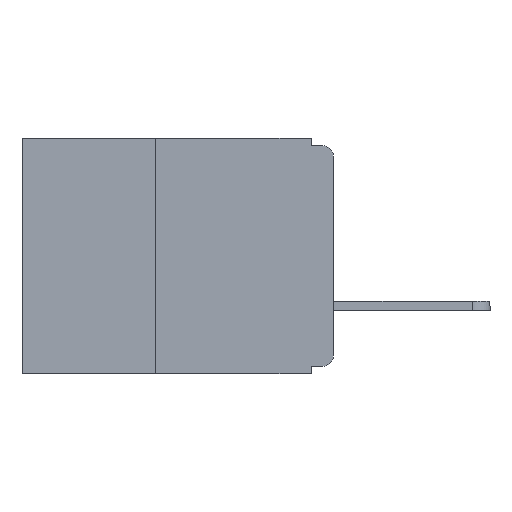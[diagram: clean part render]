
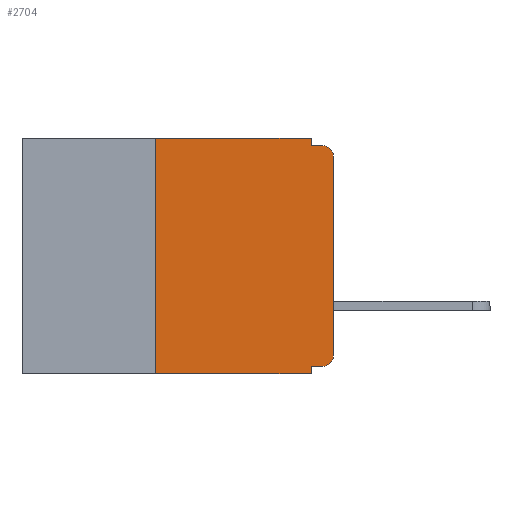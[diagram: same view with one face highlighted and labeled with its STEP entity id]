
A CAD part, left-side view. The second image highlights one B-rep face of the part: STEP entity #2704.
In plain terms, the highlighted planar face has unit normal (-1, 0, 0).
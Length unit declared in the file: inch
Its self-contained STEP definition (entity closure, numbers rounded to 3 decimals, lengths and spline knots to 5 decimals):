
#393 = ORIENTED_EDGE ( 'NONE', *, *, #2934, .F. ) ;
#670 = CARTESIAN_POINT ( 'NONE',  ( 0., 0., -0.01 ) ) ;
#1134 = CARTESIAN_POINT ( 'NONE',  ( 0., 0.437, -0.33 ) ) ;
#1519 = LINE ( 'NONE', #21604, #22971 ) ;
#2468 = DIRECTION ( 'NONE',  ( 0., 0., -1. ) ) ;
#2632 = LINE ( 'NONE', #20486, #23436 ) ;
#2704 = ADVANCED_FACE ( 'NONE', ( #4771 ), #10518, .F. ) ;
#2796 = DIRECTION ( 'NONE',  ( 0., -1., 0. ) ) ;
#2934 = EDGE_CURVE ( 'NONE', #14700, #11044, #10099, .T. ) ;
#3012 = ORIENTED_EDGE ( 'NONE', *, *, #5833, .F. ) ;
#3144 = DIRECTION ( 'NONE',  ( -1., 0., 0. ) ) ;
#3207 = CARTESIAN_POINT ( 'NONE',  ( 0., 0.031, -0.33 ) ) ;
#3247 = CARTESIAN_POINT ( 'NONE',  ( 0., 0.031, -0.33 ) ) ;
#3608 = DIRECTION ( 'NONE',  ( 0., 0., -1. ) ) ;
#3685 = CARTESIAN_POINT ( 'NONE',  ( 0., 0.031, 0. ) ) ;
#4215 = CARTESIAN_POINT ( 'NONE',  ( 0., 0.437, 0. ) ) ;
#4442 = VECTOR ( 'NONE', #2468, 39.37008 ) ;
#4647 = ORIENTED_EDGE ( 'NONE', *, *, #9009, .F. ) ;
#4750 = EDGE_CURVE ( 'NONE', #20204, #13691, #24163, .T. ) ;
#4771 = FACE_OUTER_BOUND ( 'NONE', #12851, .T. ) ;
#4803 = AXIS2_PLACEMENT_3D ( 'NONE', #15691, #3144, #17779 ) ;
#4807 = LINE ( 'NONE', #1134, #20767 ) ;
#4853 = VECTOR ( 'NONE', #2796, 39.37008 ) ;
#5833 = EDGE_CURVE ( 'NONE', #7580, #12090, #25761, .T. ) ;
#6058 = CARTESIAN_POINT ( 'NONE',  ( 0., 0.25, 0. ) ) ;
#6938 = EDGE_CURVE ( 'NONE', #25751, #11863, #2632, .T. ) ;
#7128 = DIRECTION ( 'NONE',  ( 0., -1., 0. ) ) ;
#7425 = LINE ( 'NONE', #24303, #12403 ) ;
#7580 = VERTEX_POINT ( 'NONE', #18480 ) ;
#7639 = ORIENTED_EDGE ( 'NONE', *, *, #6938, .F. ) ;
#8133 = AXIS2_PLACEMENT_3D ( 'NONE', #18391, #18327, #18323 ) ;
#8964 = ORIENTED_EDGE ( 'NONE', *, *, #17794, .T. ) ;
#9009 = EDGE_CURVE ( 'NONE', #12090, #13691, #21423, .T. ) ;
#9742 = DIRECTION ( 'NONE',  ( 0., 0., 1. ) ) ;
#10099 = LINE ( 'NONE', #3207, #4442 ) ;
#10230 = DIRECTION ( 'NONE',  ( 0., 0., 1. ) ) ;
#10518 = PLANE ( 'NONE',  #23278 ) ;
#10558 = CARTESIAN_POINT ( 'NONE',  ( 0., 0.25, -0.33 ) ) ;
#11044 = VERTEX_POINT ( 'NONE', #3247 ) ;
#11780 = CARTESIAN_POINT ( 'NONE',  ( 0., 0., 0. ) ) ;
#11863 = VERTEX_POINT ( 'NONE', #6058 ) ;
#12090 = VERTEX_POINT ( 'NONE', #20936 ) ;
#12304 = EDGE_CURVE ( 'NONE', #11863, #7580, #1519, .T. ) ;
#12403 = VECTOR ( 'NONE', #26367, 39.37008 ) ;
#12510 = EDGE_CURVE ( 'NONE', #17296, #14700, #7425, .T. ) ;
#12851 = EDGE_LOOP ( 'NONE', ( #24116, #19972, #4647, #3012, #17442, #7639, #8964, #393, #17760, #23195 ) ) ;
#13691 = VERTEX_POINT ( 'NONE', #20226 ) ;
#14700 = VERTEX_POINT ( 'NONE', #21886 ) ;
#15691 = CARTESIAN_POINT ( 'NONE',  ( 0., 0.015, -0.305 ) ) ;
#17296 = VERTEX_POINT ( 'NONE', #20790 ) ;
#17442 = ORIENTED_EDGE ( 'NONE', *, *, #12304, .F. ) ;
#17759 = EDGE_CURVE ( 'NONE', #17296, #26332, #21386, .T. ) ;
#17760 = ORIENTED_EDGE ( 'NONE', *, *, #12510, .F. ) ;
#17779 = DIRECTION ( 'NONE',  ( 0., 0., -1. ) ) ;
#17794 = EDGE_CURVE ( 'NONE', #25751, #11044, #4807, .T. ) ;
#17869 = DIRECTION ( 'NONE',  ( 0., -1., 0. ) ) ;
#18323 = DIRECTION ( 'NONE',  ( 0., 0., -1. ) ) ;
#18327 = DIRECTION ( 'NONE',  ( -1., 0., 0. ) ) ;
#18391 = CARTESIAN_POINT ( 'NONE',  ( 0., 0.015, -0.025 ) ) ;
#18447 = VECTOR ( 'NONE', #9742, 39.37008 ) ;
#18480 = CARTESIAN_POINT ( 'NONE',  ( 0., 0.031, 0. ) ) ;
#19667 = VECTOR ( 'NONE', #3608, 39.37008 ) ;
#19972 = ORIENTED_EDGE ( 'NONE', *, *, #4750, .T. ) ;
#20204 = VERTEX_POINT ( 'NONE', #26069 ) ;
#20226 = CARTESIAN_POINT ( 'NONE',  ( 0., 0.015, -0.01 ) ) ;
#20486 = CARTESIAN_POINT ( 'NONE',  ( 0., 0.25, -0.33 ) ) ;
#20767 = VECTOR ( 'NONE', #17869, 39.37008 ) ;
#20790 = CARTESIAN_POINT ( 'NONE',  ( 0., 0.015, -0.32 ) ) ;
#20936 = CARTESIAN_POINT ( 'NONE',  ( 0., 0.031, -0.01 ) ) ;
#21386 = CIRCLE ( 'NONE', #4803, 0.015 ) ;
#21423 = LINE ( 'NONE', #670, #4853 ) ;
#21604 = CARTESIAN_POINT ( 'NONE',  ( 0., 0.437, 0. ) ) ;
#21886 = CARTESIAN_POINT ( 'NONE',  ( 0., 0.031, -0.32 ) ) ;
#22971 = VECTOR ( 'NONE', #7128, 39.37008 ) ;
#23076 = CARTESIAN_POINT ( 'NONE',  ( 0., 0., -0.305 ) ) ;
#23115 = DIRECTION ( 'NONE',  ( 0., 0., -1. ) ) ;
#23195 = ORIENTED_EDGE ( 'NONE', *, *, #17759, .T. ) ;
#23241 = DIRECTION ( 'NONE',  ( 1., 0., 0. ) ) ;
#23278 = AXIS2_PLACEMENT_3D ( 'NONE', #4215, #23241, #23115 ) ;
#23436 = VECTOR ( 'NONE', #10230, 39.37008 ) ;
#23875 = LINE ( 'NONE', #11780, #18447 ) ;
#24116 = ORIENTED_EDGE ( 'NONE', *, *, #26610, .T. ) ;
#24163 = CIRCLE ( 'NONE', #8133, 0.015 ) ;
#24303 = CARTESIAN_POINT ( 'NONE',  ( 0., 0., -0.32 ) ) ;
#25751 = VERTEX_POINT ( 'NONE', #10558 ) ;
#25761 = LINE ( 'NONE', #3685, #19667 ) ;
#26069 = CARTESIAN_POINT ( 'NONE',  ( 0., 0., -0.025 ) ) ;
#26332 = VERTEX_POINT ( 'NONE', #23076 ) ;
#26367 = DIRECTION ( 'NONE',  ( 0., 1., 0. ) ) ;
#26610 = EDGE_CURVE ( 'NONE', #26332, #20204, #23875, .T. ) ;
